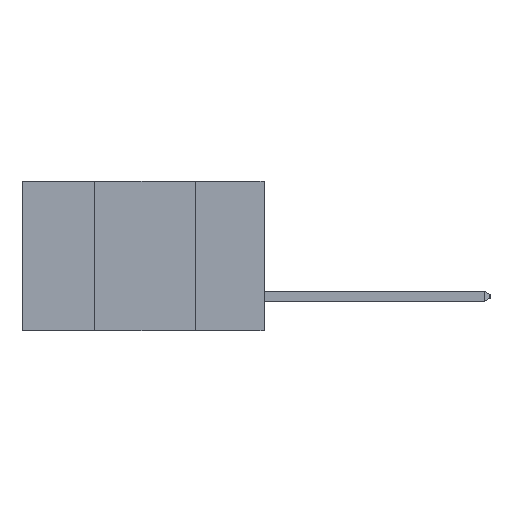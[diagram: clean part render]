
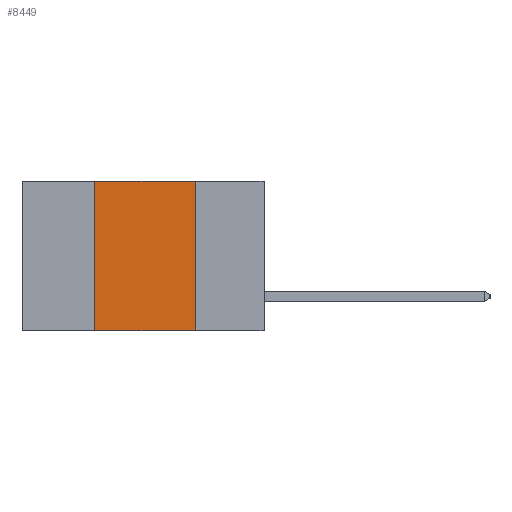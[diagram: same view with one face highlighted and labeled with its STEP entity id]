
A CAD part, left-side view. The second image highlights one B-rep face of the part: STEP entity #8449.
In plain terms, the highlighted planar face has unit normal (-1, 0, 0).
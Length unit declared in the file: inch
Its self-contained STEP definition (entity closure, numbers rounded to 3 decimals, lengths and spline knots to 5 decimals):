
#704 = CARTESIAN_POINT ( 'NONE',  ( 0., 0.6, -0.37 ) ) ;
#2355 = PLANE ( 'NONE',  #19312 ) ;
#3103 = EDGE_CURVE ( 'NONE', #20044, #24907, #10876, .T. ) ;
#4374 = CARTESIAN_POINT ( 'NONE',  ( 0., 0.6, 0. ) ) ;
#4446 = VERTEX_POINT ( 'NONE', #20226 ) ;
#5170 = CARTESIAN_POINT ( 'NONE',  ( 0., 0.17, 0. ) ) ;
#5235 = CARTESIAN_POINT ( 'NONE',  ( 0., 0.42, -0.37 ) ) ;
#5397 = CARTESIAN_POINT ( 'NONE',  ( 0., 0.42, 0. ) ) ;
#5736 = VECTOR ( 'NONE', #17573, 39.37008 ) ;
#6443 = DIRECTION ( 'NONE',  ( 1., 0., 0. ) ) ;
#6532 = VECTOR ( 'NONE', #6820, 39.37008 ) ;
#6820 = DIRECTION ( 'NONE',  ( 0., -1., 0. ) ) ;
#7272 = FACE_OUTER_BOUND ( 'NONE', #17376, .T. ) ;
#7377 = VECTOR ( 'NONE', #15261, 39.37008 ) ;
#8449 = ADVANCED_FACE ( 'NONE', ( #7272 ), #2355, .F. ) ;
#10876 = LINE ( 'NONE', #5397, #16309 ) ;
#11649 = DIRECTION ( 'NONE',  ( 0., 0., 1. ) ) ;
#11873 = EDGE_CURVE ( 'NONE', #20044, #19535, #16803, .T. ) ;
#12827 = LINE ( 'NONE', #13210, #7377 ) ;
#13210 = CARTESIAN_POINT ( 'NONE',  ( 0., 0.6, 0. ) ) ;
#13871 = ORIENTED_EDGE ( 'NONE', *, *, #3103, .F. ) ;
#14536 = ORIENTED_EDGE ( 'NONE', *, *, #14793, .F. ) ;
#14793 = EDGE_CURVE ( 'NONE', #24907, #4446, #12827, .T. ) ;
#15261 = DIRECTION ( 'NONE',  ( 0., -1., 0. ) ) ;
#15481 = EDGE_CURVE ( 'NONE', #4446, #19535, #22090, .T. ) ;
#16309 = VECTOR ( 'NONE', #11649, 39.37008 ) ;
#16803 = LINE ( 'NONE', #704, #6532 ) ;
#17376 = EDGE_LOOP ( 'NONE', ( #25323, #14536, #13871, #22281 ) ) ;
#17573 = DIRECTION ( 'NONE',  ( 0., 0., -1. ) ) ;
#19312 = AXIS2_PLACEMENT_3D ( 'NONE', #4374, #6443, #20821 ) ;
#19535 = VERTEX_POINT ( 'NONE', #21669 ) ;
#20044 = VERTEX_POINT ( 'NONE', #5235 ) ;
#20226 = CARTESIAN_POINT ( 'NONE',  ( 0., 0.17, 0. ) ) ;
#20821 = DIRECTION ( 'NONE',  ( 0., 0., -1. ) ) ;
#21669 = CARTESIAN_POINT ( 'NONE',  ( 0., 0.17, -0.37 ) ) ;
#22090 = LINE ( 'NONE', #5170, #5736 ) ;
#22281 = ORIENTED_EDGE ( 'NONE', *, *, #11873, .T. ) ;
#22310 = CARTESIAN_POINT ( 'NONE',  ( 0., 0.42, 0. ) ) ;
#24907 = VERTEX_POINT ( 'NONE', #22310 ) ;
#25323 = ORIENTED_EDGE ( 'NONE', *, *, #15481, .F. ) ;
